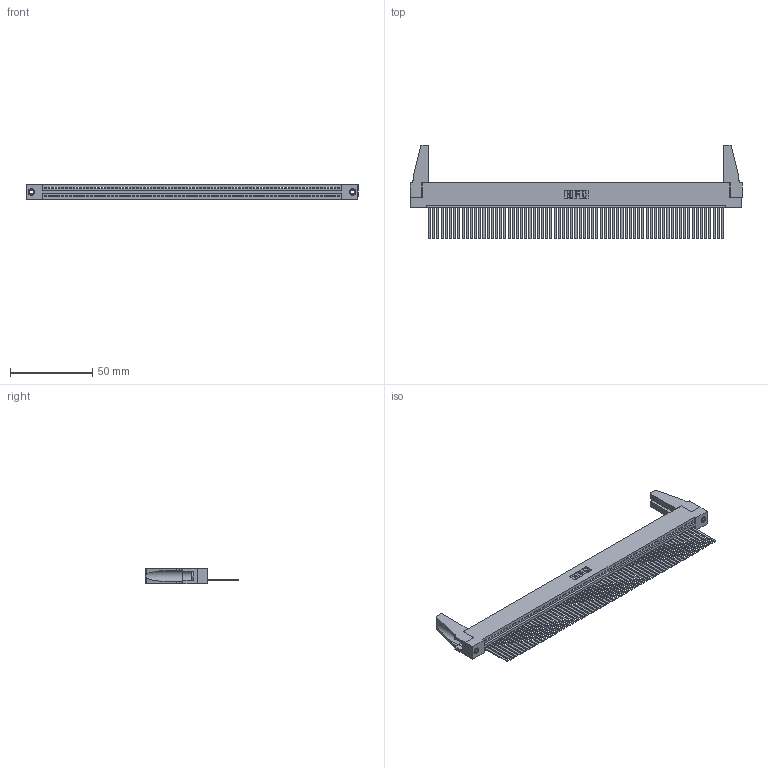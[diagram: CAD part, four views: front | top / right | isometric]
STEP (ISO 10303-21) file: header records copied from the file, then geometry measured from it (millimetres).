
FILE_DESCRIPTION (( 'STEP AP203' ), '1' );
FILE_NAME ('395-071-544-188.STEP', '2019-10-26T06:27:35', ( '' ), ( '' ), 'SwSTEP 2.0', 'SolidWorks 2016', '' );
FILE_SCHEMA (( 'CONFIG_CONTROL_DESIGN' ));
Length unit declared in the file: inch
Products named in the file (5): 395-071-544-188; 345-250-001_345-250-001-102; 345 Part_Flush Mounting Lugs - 0.156 Dia-TH; 345-292-001_345-293-144; 345-220-078_345-220-088
Assembly tree (76 placements, depth 2):
  395-071-544-188
    345 Part_Flush Mounting Lugs - 0.156 Dia-TH
    345-292-001_345-293-144  x71
    345-250-001_345-250-001-102  x2
    345-220-078_345-220-088  x2
Bounding box: 201.57 x 56.82 x 9.4 mm (x, y, z)
Volume: 23458.1 mm3; surface area: 32843.3 mm2
Topology: 76 solids, 76 shells, 3942 faces, 11873 edges, 7810 vertices
Faces by surface type: plane 2708, cylinder 1218, cone 12, torus 4
Entity records: 51496 total; most frequent: CARTESIAN_POINT 8907, ORIENTED_EDGE 8872, DIRECTION 7742, EDGE_CURVE 4436, LINE 3982, VECTOR 3982, VERTEX_POINT 2950, AXIS2_PLACEMENT_3D 1880
